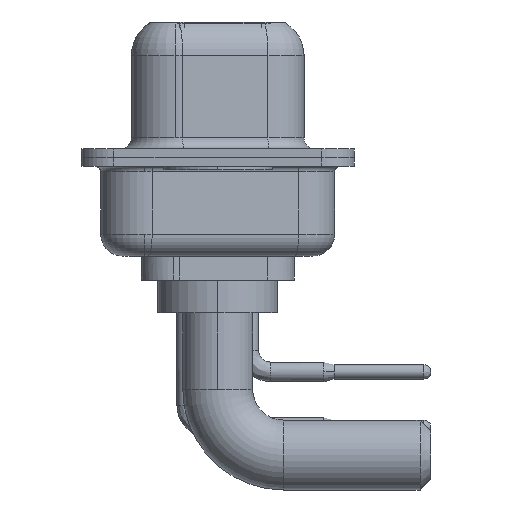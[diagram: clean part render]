
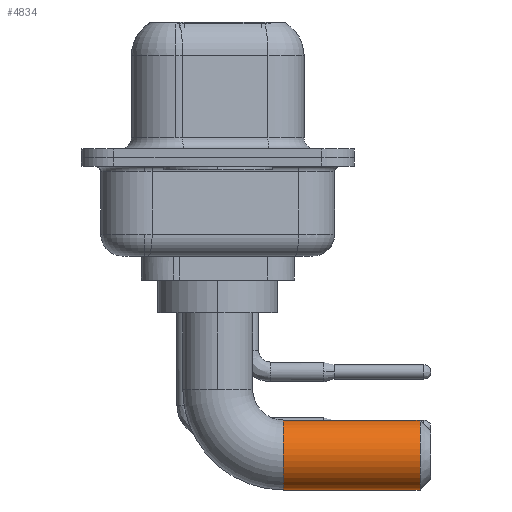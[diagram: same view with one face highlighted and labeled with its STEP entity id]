
A CAD part, left-side view. The second image highlights one B-rep face of the part: STEP entity #4834.
In plain terms, the highlighted cylindrical face has radius 1.6 mm (diameter 3.2 mm), a partial arc.
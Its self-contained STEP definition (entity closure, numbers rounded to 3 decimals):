
#249 = FACE_OUTER_BOUND ( 'NONE', #16439, .T. ) ;
#398 = AXIS2_PLACEMENT_3D ( 'NONE', #1199, #10903, #6888 ) ;
#1199 = CARTESIAN_POINT ( 'NONE',  ( 0., -9.25, -6.5 ) ) ;
#1310 = DIRECTION ( 'NONE',  ( -1., 0., 0. ) ) ;
#1399 = CARTESIAN_POINT ( 'NONE',  ( 0., -3., -6.5 ) ) ;
#3228 = DIRECTION ( 'NONE',  ( 0., -1., 0. ) ) ;
#4270 = CARTESIAN_POINT ( 'NONE',  ( 0., -3., -6.5 ) ) ;
#4512 = VERTEX_POINT ( 'NONE', #5785 ) ;
#4548 = DIRECTION ( 'NONE',  ( 0., -1., 0. ) ) ;
#4697 = EDGE_CURVE ( 'NONE', #14052, #4512, #5675, .T. ) ;
#4834 = ADVANCED_FACE ( 'NONE', ( #249 ), #11360, .T. ) ;
#5675 = CIRCLE ( 'NONE', #398, 1.6 ) ;
#5785 = CARTESIAN_POINT ( 'NONE',  ( 0., -9.25, -4.9 ) ) ;
#6290 = CARTESIAN_POINT ( 'NONE',  ( 0., -3., -8.1 ) ) ;
#6324 = ORIENTED_EDGE ( 'NONE', *, *, #11690, .T. ) ;
#6490 = CIRCLE ( 'NONE', #14802, 1.6 ) ;
#6888 = DIRECTION ( 'NONE',  ( 0., 0., -1. ) ) ;
#7098 = VECTOR ( 'NONE', #16793, 1000. ) ;
#7432 = LINE ( 'NONE', #7525, #18059 ) ;
#7525 = CARTESIAN_POINT ( 'NONE',  ( 0., -3., -8.1 ) ) ;
#7735 = CARTESIAN_POINT ( 'NONE',  ( 0., -9.25, -8.1 ) ) ;
#8133 = CARTESIAN_POINT ( 'NONE',  ( 0., -3., -4.9 ) ) ;
#8517 = ORIENTED_EDGE ( 'NONE', *, *, #12041, .F. ) ;
#9390 = EDGE_CURVE ( 'NONE', #14886, #14052, #7432, .T. ) ;
#9820 = LINE ( 'NONE', #8133, #7098 ) ;
#10903 = DIRECTION ( 'NONE',  ( 0., 1., 0. ) ) ;
#11360 = CYLINDRICAL_SURFACE ( 'NONE', #14120, 1.6 ) ;
#11445 = DIRECTION ( 'NONE',  ( 0., 0., -1. ) ) ;
#11690 = EDGE_CURVE ( 'NONE', #15654, #14886, #6490, .T. ) ;
#11962 = ORIENTED_EDGE ( 'NONE', *, *, #9390, .T. ) ;
#12041 = EDGE_CURVE ( 'NONE', #15654, #4512, #9820, .T. ) ;
#14052 = VERTEX_POINT ( 'NONE', #7735 ) ;
#14120 = AXIS2_PLACEMENT_3D ( 'NONE', #4270, #4548, #11445 ) ;
#14802 = AXIS2_PLACEMENT_3D ( 'NONE', #1399, #18350, #1310 ) ;
#14886 = VERTEX_POINT ( 'NONE', #6290 ) ;
#15654 = VERTEX_POINT ( 'NONE', #15659 ) ;
#15659 = CARTESIAN_POINT ( 'NONE',  ( 0., -3., -4.9 ) ) ;
#16439 = EDGE_LOOP ( 'NONE', ( #8517, #6324, #11962, #17311 ) ) ;
#16793 = DIRECTION ( 'NONE',  ( 0., -1., 0. ) ) ;
#17311 = ORIENTED_EDGE ( 'NONE', *, *, #4697, .T. ) ;
#18059 = VECTOR ( 'NONE', #3228, 1000. ) ;
#18350 = DIRECTION ( 'NONE',  ( 0., -1., 0. ) ) ;
